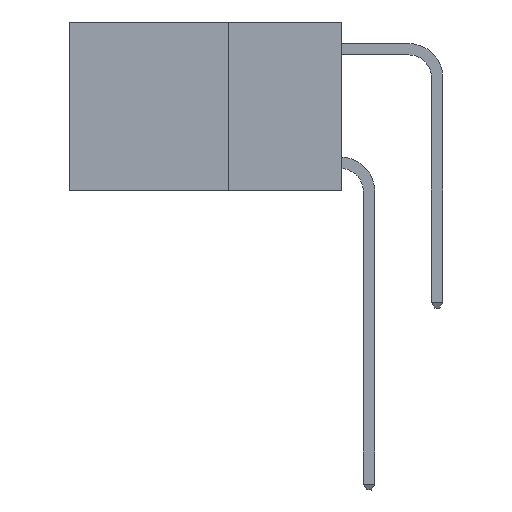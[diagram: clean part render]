
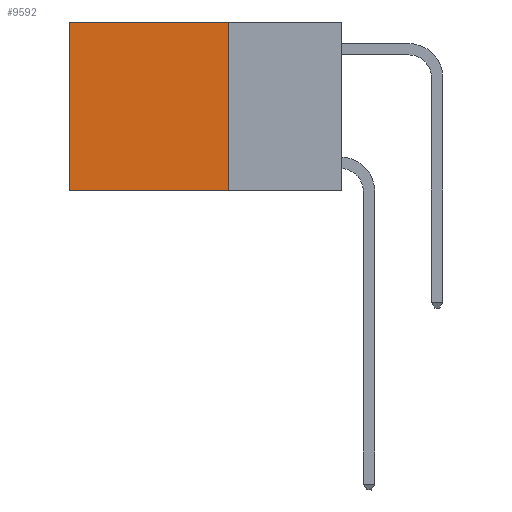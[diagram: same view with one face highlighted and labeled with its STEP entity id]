
A CAD part, left-side view. The second image highlights one B-rep face of the part: STEP entity #9592.
In plain terms, the highlighted planar face has unit normal (-1, 0, 0).
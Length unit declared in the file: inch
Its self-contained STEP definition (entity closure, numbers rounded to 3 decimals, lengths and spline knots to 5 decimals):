
#413 = ORIENTED_EDGE ( 'NONE', *, *, #1808, .F. ) ;
#1226 = EDGE_CURVE ( 'NONE', #6255, #2504, #8153, .T. ) ;
#1778 = CARTESIAN_POINT ( 'NONE',  ( 0.2625, 0.25, 0. ) ) ;
#1808 = EDGE_CURVE ( 'NONE', #14527, #12717, #4057, .T. ) ;
#2054 = CARTESIAN_POINT ( 'NONE',  ( 0.2625, 0.25, -0.37 ) ) ;
#2415 = EDGE_CURVE ( 'NONE', #14527, #6255, #14006, .T. ) ;
#2504 = VERTEX_POINT ( 'NONE', #8314 ) ;
#2832 = VECTOR ( 'NONE', #15503, 39.37008 ) ;
#3300 = VECTOR ( 'NONE', #14013, 39.37008 ) ;
#3782 = ORIENTED_EDGE ( 'NONE', *, *, #1226, .T. ) ;
#3838 = ORIENTED_EDGE ( 'NONE', *, *, #15238, .F. ) ;
#4057 = LINE ( 'NONE', #5180, #12842 ) ;
#5129 = VECTOR ( 'NONE', #10332, 39.37008 ) ;
#5180 = CARTESIAN_POINT ( 'NONE',  ( 0.2625, 0.25, 0. ) ) ;
#6255 = VERTEX_POINT ( 'NONE', #12318 ) ;
#6827 = CARTESIAN_POINT ( 'NONE',  ( 0.2625, 0.25, 0. ) ) ;
#7452 = PLANE ( 'NONE',  #9697 ) ;
#8153 = LINE ( 'NONE', #12982, #3300 ) ;
#8314 = CARTESIAN_POINT ( 'NONE',  ( 0.2625, 0.6, -0.37 ) ) ;
#8428 = LINE ( 'NONE', #2054, #2832 ) ;
#8502 = CARTESIAN_POINT ( 'NONE',  ( 0.2625, 0.25, 0. ) ) ;
#8730 = DIRECTION ( 'NONE',  ( 0., 0., -1. ) ) ;
#8910 = CARTESIAN_POINT ( 'NONE',  ( 0.2625, 0.25, -0.37 ) ) ;
#9592 = ADVANCED_FACE ( 'NONE', ( #12286 ), #7452, .F. ) ;
#9607 = ORIENTED_EDGE ( 'NONE', *, *, #2415, .T. ) ;
#9697 = AXIS2_PLACEMENT_3D ( 'NONE', #8502, #11079, #8730 ) ;
#10332 = DIRECTION ( 'NONE',  ( 0., 1., 0. ) ) ;
#11079 = DIRECTION ( 'NONE',  ( 1., 0., 0. ) ) ;
#11661 = EDGE_LOOP ( 'NONE', ( #3782, #3838, #413, #9607 ) ) ;
#12286 = FACE_OUTER_BOUND ( 'NONE', #11661, .T. ) ;
#12318 = CARTESIAN_POINT ( 'NONE',  ( 0.2625, 0.6, 0. ) ) ;
#12717 = VERTEX_POINT ( 'NONE', #8910 ) ;
#12842 = VECTOR ( 'NONE', #15164, 39.37008 ) ;
#12982 = CARTESIAN_POINT ( 'NONE',  ( 0.2625, 0.6, 0. ) ) ;
#14006 = LINE ( 'NONE', #1778, #5129 ) ;
#14013 = DIRECTION ( 'NONE',  ( 0., 0., -1. ) ) ;
#14527 = VERTEX_POINT ( 'NONE', #6827 ) ;
#15164 = DIRECTION ( 'NONE',  ( 0., 0., -1. ) ) ;
#15238 = EDGE_CURVE ( 'NONE', #12717, #2504, #8428, .T. ) ;
#15503 = DIRECTION ( 'NONE',  ( 0., 1., 0. ) ) ;
